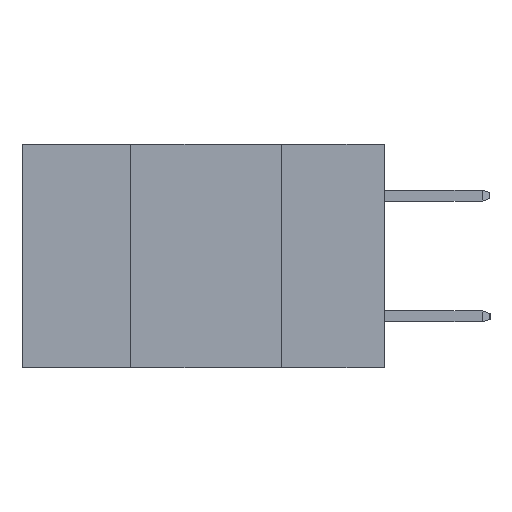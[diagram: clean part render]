
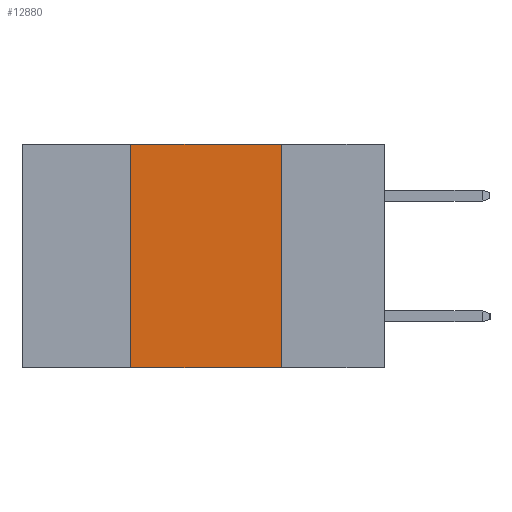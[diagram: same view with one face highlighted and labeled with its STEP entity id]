
A CAD part, left-side view. The second image highlights one B-rep face of the part: STEP entity #12880.
In plain terms, the highlighted planar face has unit normal (-1, 0, 0).
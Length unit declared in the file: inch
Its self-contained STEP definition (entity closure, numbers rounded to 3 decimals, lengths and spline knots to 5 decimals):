
#76 = EDGE_LOOP ( 'NONE', ( #10608, #9971, #15574, #853 ) ) ;
#291 = LINE ( 'NONE', #10464, #6229 ) ;
#545 = CARTESIAN_POINT ( 'NONE',  ( 0., 0.17, -0.37 ) ) ;
#853 = ORIENTED_EDGE ( 'NONE', *, *, #11101, .T. ) ;
#1207 = VERTEX_POINT ( 'NONE', #5692 ) ;
#1233 = CARTESIAN_POINT ( 'NONE',  ( 0., 0.42, -0.37 ) ) ;
#1480 = CARTESIAN_POINT ( 'NONE',  ( 0., 0.17, -0.37 ) ) ;
#1581 = DIRECTION ( 'NONE',  ( 0., -1., 0. ) ) ;
#2318 = CARTESIAN_POINT ( 'NONE',  ( 0., 0.6, 0. ) ) ;
#3575 = DIRECTION ( 'NONE',  ( 0., 0., -1. ) ) ;
#3746 = VERTEX_POINT ( 'NONE', #1480 ) ;
#3787 = CARTESIAN_POINT ( 'NONE',  ( 0., 0.42, -0.37 ) ) ;
#3941 = CARTESIAN_POINT ( 'NONE',  ( 0., 0.42, 0. ) ) ;
#4490 = VECTOR ( 'NONE', #15829, 39.37008 ) ;
#5692 = CARTESIAN_POINT ( 'NONE',  ( 0., 0.17, 0. ) ) ;
#6229 = VECTOR ( 'NONE', #1581, 39.37008 ) ;
#6596 = DIRECTION ( 'NONE',  ( 0., -1., 0. ) ) ;
#6947 = EDGE_CURVE ( 'NONE', #7631, #11038, #13689, .T. ) ;
#7631 = VERTEX_POINT ( 'NONE', #1233 ) ;
#8013 = VECTOR ( 'NONE', #6596, 39.37008 ) ;
#9971 = ORIENTED_EDGE ( 'NONE', *, *, #10503, .F. ) ;
#10308 = VECTOR ( 'NONE', #15251, 39.37008 ) ;
#10394 = CARTESIAN_POINT ( 'NONE',  ( 0., 0.6, -0.37 ) ) ;
#10464 = CARTESIAN_POINT ( 'NONE',  ( 0., 0.6, 0. ) ) ;
#10503 = EDGE_CURVE ( 'NONE', #11038, #1207, #291, .T. ) ;
#10608 = ORIENTED_EDGE ( 'NONE', *, *, #14762, .F. ) ;
#11038 = VERTEX_POINT ( 'NONE', #3941 ) ;
#11101 = EDGE_CURVE ( 'NONE', #7631, #3746, #11408, .T. ) ;
#11223 = DIRECTION ( 'NONE',  ( 1., 0., 0. ) ) ;
#11285 = LINE ( 'NONE', #545, #4490 ) ;
#11408 = LINE ( 'NONE', #10394, #8013 ) ;
#11736 = FACE_OUTER_BOUND ( 'NONE', #76, .T. ) ;
#12880 = ADVANCED_FACE ( 'NONE', ( #11736 ), #16262, .F. ) ;
#13689 = LINE ( 'NONE', #3787, #10308 ) ;
#14762 = EDGE_CURVE ( 'NONE', #1207, #3746, #11285, .T. ) ;
#15251 = DIRECTION ( 'NONE',  ( 0., 0., 1. ) ) ;
#15508 = AXIS2_PLACEMENT_3D ( 'NONE', #2318, #11223, #3575 ) ;
#15574 = ORIENTED_EDGE ( 'NONE', *, *, #6947, .F. ) ;
#15829 = DIRECTION ( 'NONE',  ( 0., 0., -1. ) ) ;
#16262 = PLANE ( 'NONE',  #15508 ) ;
